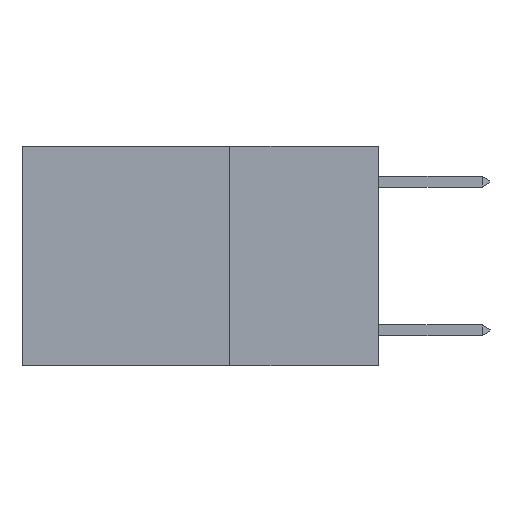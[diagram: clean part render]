
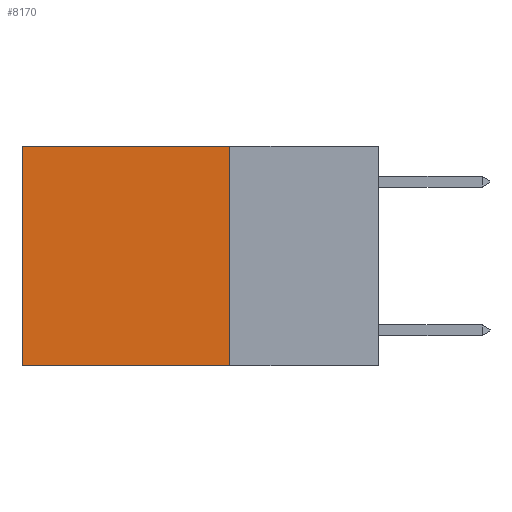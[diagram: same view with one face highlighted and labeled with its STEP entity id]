
A CAD part, left-side view. The second image highlights one B-rep face of the part: STEP entity #8170.
In plain terms, the highlighted planar face has unit normal (-1, 0, 0).
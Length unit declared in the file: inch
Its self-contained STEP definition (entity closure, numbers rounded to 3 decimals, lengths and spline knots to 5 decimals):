
#178 = VERTEX_POINT ( 'NONE', #1317 ) ;
#292 = CARTESIAN_POINT ( 'NONE',  ( 0.2625, 0.6, 0. ) ) ;
#930 = CARTESIAN_POINT ( 'NONE',  ( 0.2625, 0.6, -0.37 ) ) ;
#1179 = DIRECTION ( 'NONE',  ( 0., 0., -1. ) ) ;
#1229 = ORIENTED_EDGE ( 'NONE', *, *, #5475, .F. ) ;
#1317 = CARTESIAN_POINT ( 'NONE',  ( 0.2625, 0.6, 0. ) ) ;
#1461 = LINE ( 'NONE', #7687, #5521 ) ;
#1733 = FACE_OUTER_BOUND ( 'NONE', #6672, .T. ) ;
#1880 = VECTOR ( 'NONE', #1179, 39.37008 ) ;
#1915 = VERTEX_POINT ( 'NONE', #930 ) ;
#2180 = LINE ( 'NONE', #292, #1880 ) ;
#2239 = EDGE_CURVE ( 'NONE', #10013, #5734, #7019, .T. ) ;
#2776 = DIRECTION ( 'NONE',  ( 0., 0., -1. ) ) ;
#3537 = LINE ( 'NONE', #4926, #7345 ) ;
#3776 = PLANE ( 'NONE',  #7230 ) ;
#4558 = DIRECTION ( 'NONE',  ( 0., 0., -1. ) ) ;
#4633 = ORIENTED_EDGE ( 'NONE', *, *, #2239, .F. ) ;
#4695 = EDGE_CURVE ( 'NONE', #10013, #178, #1461, .T. ) ;
#4926 = CARTESIAN_POINT ( 'NONE',  ( 0.2625, 0.25, -0.37 ) ) ;
#5414 = CARTESIAN_POINT ( 'NONE',  ( 0.2625, 0.25, 0. ) ) ;
#5475 = EDGE_CURVE ( 'NONE', #5734, #1915, #3537, .T. ) ;
#5521 = VECTOR ( 'NONE', #8398, 39.37008 ) ;
#5734 = VERTEX_POINT ( 'NONE', #9562 ) ;
#6063 = CARTESIAN_POINT ( 'NONE',  ( 0.2625, 0.25, 0. ) ) ;
#6672 = EDGE_LOOP ( 'NONE', ( #9869, #1229, #4633, #9769 ) ) ;
#6780 = VECTOR ( 'NONE', #2776, 39.37008 ) ;
#7019 = LINE ( 'NONE', #5414, #6780 ) ;
#7230 = AXIS2_PLACEMENT_3D ( 'NONE', #6063, #8983, #4558 ) ;
#7345 = VECTOR ( 'NONE', #9320, 39.37008 ) ;
#7687 = CARTESIAN_POINT ( 'NONE',  ( 0.2625, 0.25, 0. ) ) ;
#8170 = ADVANCED_FACE ( 'NONE', ( #1733 ), #3776, .F. ) ;
#8398 = DIRECTION ( 'NONE',  ( 0., 1., 0. ) ) ;
#8432 = EDGE_CURVE ( 'NONE', #178, #1915, #2180, .T. ) ;
#8711 = CARTESIAN_POINT ( 'NONE',  ( 0.2625, 0.25, 0. ) ) ;
#8983 = DIRECTION ( 'NONE',  ( 1., 0., 0. ) ) ;
#9320 = DIRECTION ( 'NONE',  ( 0., 1., 0. ) ) ;
#9562 = CARTESIAN_POINT ( 'NONE',  ( 0.2625, 0.25, -0.37 ) ) ;
#9769 = ORIENTED_EDGE ( 'NONE', *, *, #4695, .T. ) ;
#9869 = ORIENTED_EDGE ( 'NONE', *, *, #8432, .T. ) ;
#10013 = VERTEX_POINT ( 'NONE', #8711 ) ;
